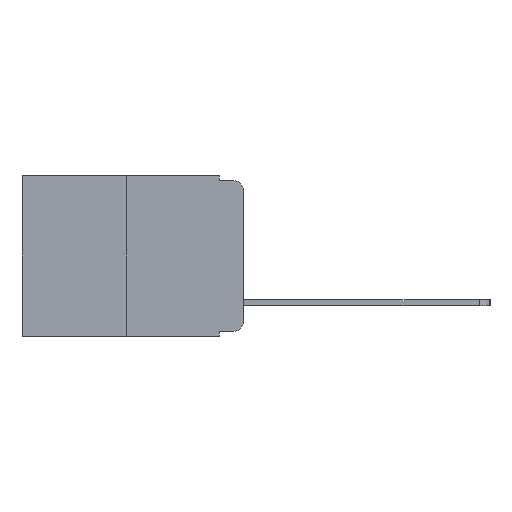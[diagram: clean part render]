
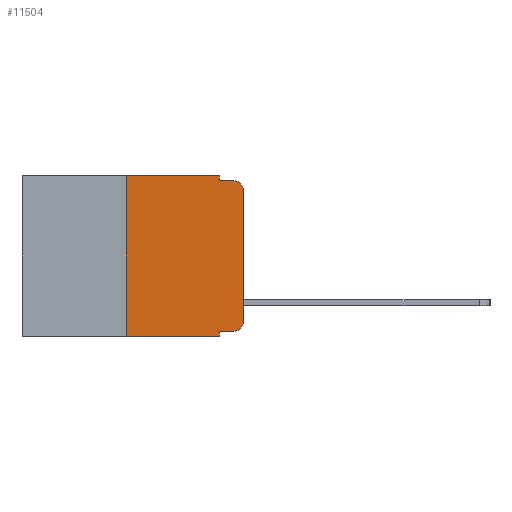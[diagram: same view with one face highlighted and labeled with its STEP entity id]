
A CAD part, left-side view. The second image highlights one B-rep face of the part: STEP entity #11504.
In plain terms, the highlighted planar face has unit normal (-1, 0, 0).
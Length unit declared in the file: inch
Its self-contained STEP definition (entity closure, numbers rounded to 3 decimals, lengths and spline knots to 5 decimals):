
#165 = CARTESIAN_POINT ( 'NONE',  ( 0., 0.051, -0.01 ) ) ;
#251 = FACE_OUTER_BOUND ( 'NONE', #8107, .T. ) ;
#348 = DIRECTION ( 'NONE',  ( 0., 0., -1. ) ) ;
#658 = CARTESIAN_POINT ( 'NONE',  ( 0., 0.02, -0.03 ) ) ;
#733 = EDGE_CURVE ( 'NONE', #3529, #14714, #11834, .T. ) ;
#1048 = LINE ( 'NONE', #7211, #3935 ) ;
#1336 = EDGE_CURVE ( 'NONE', #4087, #7202, #3976, .T. ) ;
#1914 = DIRECTION ( 'NONE',  ( 0., 0., -1. ) ) ;
#2253 = LINE ( 'NONE', #10771, #9208 ) ;
#2286 = VECTOR ( 'NONE', #6323, 39.37008 ) ;
#2373 = VERTEX_POINT ( 'NONE', #6372 ) ;
#2398 = EDGE_CURVE ( 'NONE', #2373, #13694, #10922, .T. ) ;
#2479 = DIRECTION ( 'NONE',  ( -1., 0., 0. ) ) ;
#2658 = LINE ( 'NONE', #165, #2286 ) ;
#2952 = LINE ( 'NONE', #10553, #15441 ) ;
#3006 = EDGE_CURVE ( 'NONE', #4087, #3529, #2253, .T. ) ;
#3211 = DIRECTION ( 'NONE',  ( 0., 0., 1. ) ) ;
#3320 = CARTESIAN_POINT ( 'NONE',  ( 0., 0.02, -0.313 ) ) ;
#3529 = VERTEX_POINT ( 'NONE', #15168 ) ;
#3606 = CARTESIAN_POINT ( 'NONE',  ( 0., 0.473, 0. ) ) ;
#3665 = DIRECTION ( 'NONE',  ( 1., 0., 0. ) ) ;
#3935 = VECTOR ( 'NONE', #14453, 39.37008 ) ;
#3976 = LINE ( 'NONE', #7918, #6478 ) ;
#4063 = DIRECTION ( 'NONE',  ( 0., -1., 0. ) ) ;
#4087 = VERTEX_POINT ( 'NONE', #15313 ) ;
#4422 = ORIENTED_EDGE ( 'NONE', *, *, #14665, .T. ) ;
#4661 = EDGE_CURVE ( 'NONE', #13694, #12731, #2952, .T. ) ;
#4665 = DIRECTION ( 'NONE',  ( 0., 0., -1. ) ) ;
#4782 = LINE ( 'NONE', #8588, #14043 ) ;
#4975 = ORIENTED_EDGE ( 'NONE', *, *, #733, .F. ) ;
#5312 = VECTOR ( 'NONE', #8514, 39.37008 ) ;
#6189 = LINE ( 'NONE', #10817, #15040 ) ;
#6323 = DIRECTION ( 'NONE',  ( 0., -1., 0. ) ) ;
#6372 = CARTESIAN_POINT ( 'NONE',  ( 0., 0.02, -0.333 ) ) ;
#6478 = VECTOR ( 'NONE', #4063, 39.37008 ) ;
#6936 = AXIS2_PLACEMENT_3D ( 'NONE', #3320, #2479, #348 ) ;
#7202 = VERTEX_POINT ( 'NONE', #14107 ) ;
#7211 = CARTESIAN_POINT ( 'NONE',  ( 0., 0.051, -0.333 ) ) ;
#7430 = EDGE_CURVE ( 'NONE', #14714, #12008, #4782, .T. ) ;
#7512 = ORIENTED_EDGE ( 'NONE', *, *, #13032, .F. ) ;
#7918 = CARTESIAN_POINT ( 'NONE',  ( 0., 0.473, -0.343 ) ) ;
#8107 = EDGE_LOOP ( 'NONE', ( #15473, #4422, #13486, #14970, #4975, #9443, #15554, #7512, #14511, #13588 ) ) ;
#8120 = DIRECTION ( 'NONE',  ( 0., 0., 1. ) ) ;
#8484 = CIRCLE ( 'NONE', #13907, 0.02 ) ;
#8514 = DIRECTION ( 'NONE',  ( 0., -1., 0. ) ) ;
#8546 = CARTESIAN_POINT ( 'NONE',  ( 0., 0.473, 0. ) ) ;
#8588 = CARTESIAN_POINT ( 'NONE',  ( 0., 0.051, 0. ) ) ;
#9208 = VECTOR ( 'NONE', #3211, 39.37008 ) ;
#9269 = VERTEX_POINT ( 'NONE', #14927 ) ;
#9312 = DIRECTION ( 'NONE',  ( -1., 0., 0. ) ) ;
#9443 = ORIENTED_EDGE ( 'NONE', *, *, #3006, .F. ) ;
#9619 = CARTESIAN_POINT ( 'NONE',  ( 0., 0., -0.313 ) ) ;
#9845 = CARTESIAN_POINT ( 'NONE',  ( 0., 0.051, -0.333 ) ) ;
#10248 = VERTEX_POINT ( 'NONE', #9845 ) ;
#10553 = CARTESIAN_POINT ( 'NONE',  ( 0., 0., 0. ) ) ;
#10771 = CARTESIAN_POINT ( 'NONE',  ( 0., 0.25, 0. ) ) ;
#10817 = CARTESIAN_POINT ( 'NONE',  ( 0., 0.051, 0. ) ) ;
#10922 = CIRCLE ( 'NONE', #6936, 0.02 ) ;
#11030 = PLANE ( 'NONE',  #12730 ) ;
#11445 = EDGE_CURVE ( 'NONE', #10248, #2373, #1048, .T. ) ;
#11504 = ADVANCED_FACE ( 'NONE', ( #251 ), #11030, .F. ) ;
#11834 = LINE ( 'NONE', #8546, #5312 ) ;
#12008 = VERTEX_POINT ( 'NONE', #12104 ) ;
#12104 = CARTESIAN_POINT ( 'NONE',  ( 0., 0.051, -0.01 ) ) ;
#12211 = DIRECTION ( 'NONE',  ( 0., 0., -1. ) ) ;
#12224 = DIRECTION ( 'NONE',  ( 0., 0., -1. ) ) ;
#12554 = CARTESIAN_POINT ( 'NONE',  ( 0., 0., -0.03 ) ) ;
#12730 = AXIS2_PLACEMENT_3D ( 'NONE', #3606, #3665, #12211 ) ;
#12731 = VERTEX_POINT ( 'NONE', #12554 ) ;
#12903 = CARTESIAN_POINT ( 'NONE',  ( 0., 0.051, 0. ) ) ;
#13032 = EDGE_CURVE ( 'NONE', #10248, #7202, #6189, .T. ) ;
#13486 = ORIENTED_EDGE ( 'NONE', *, *, #15077, .F. ) ;
#13588 = ORIENTED_EDGE ( 'NONE', *, *, #2398, .T. ) ;
#13694 = VERTEX_POINT ( 'NONE', #9619 ) ;
#13907 = AXIS2_PLACEMENT_3D ( 'NONE', #658, #9312, #1914 ) ;
#14043 = VECTOR ( 'NONE', #12224, 39.37008 ) ;
#14107 = CARTESIAN_POINT ( 'NONE',  ( 0., 0.051, -0.343 ) ) ;
#14453 = DIRECTION ( 'NONE',  ( 0., -1., 0. ) ) ;
#14511 = ORIENTED_EDGE ( 'NONE', *, *, #11445, .T. ) ;
#14665 = EDGE_CURVE ( 'NONE', #12731, #9269, #8484, .T. ) ;
#14714 = VERTEX_POINT ( 'NONE', #12903 ) ;
#14927 = CARTESIAN_POINT ( 'NONE',  ( 0., 0.02, -0.01 ) ) ;
#14970 = ORIENTED_EDGE ( 'NONE', *, *, #7430, .F. ) ;
#15040 = VECTOR ( 'NONE', #4665, 39.37008 ) ;
#15077 = EDGE_CURVE ( 'NONE', #12008, #9269, #2658, .T. ) ;
#15168 = CARTESIAN_POINT ( 'NONE',  ( 0., 0.25, 0. ) ) ;
#15313 = CARTESIAN_POINT ( 'NONE',  ( 0., 0.25, -0.343 ) ) ;
#15441 = VECTOR ( 'NONE', #8120, 39.37008 ) ;
#15473 = ORIENTED_EDGE ( 'NONE', *, *, #4661, .T. ) ;
#15554 = ORIENTED_EDGE ( 'NONE', *, *, #1336, .T. ) ;
